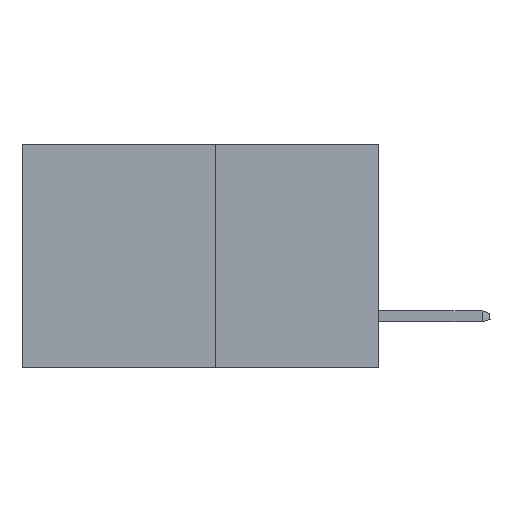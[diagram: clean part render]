
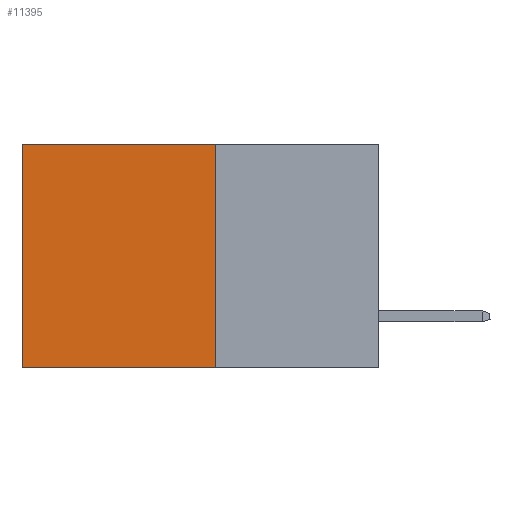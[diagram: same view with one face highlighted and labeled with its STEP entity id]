
A CAD part, left-side view. The second image highlights one B-rep face of the part: STEP entity #11395.
In plain terms, the highlighted planar face has unit normal (-1, 0, 0).
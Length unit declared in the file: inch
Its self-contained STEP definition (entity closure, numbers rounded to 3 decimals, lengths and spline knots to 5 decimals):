
#9 = DIRECTION ( 'NONE',  ( 0., 1., 0. ) ) ;
#455 = CARTESIAN_POINT ( 'NONE',  ( 0.277, 0.27, -0.37 ) ) ;
#3678 = DIRECTION ( 'NONE',  ( 0., 0., -1. ) ) ;
#4418 = LINE ( 'NONE', #22667, #19789 ) ;
#4573 = CARTESIAN_POINT ( 'NONE',  ( 0.277, 0.27, -0.37 ) ) ;
#4858 = LINE ( 'NONE', #13778, #20225 ) ;
#5919 = VECTOR ( 'NONE', #3678, 39.37008 ) ;
#6550 = EDGE_CURVE ( 'NONE', #22512, #9463, #9322, .T. ) ;
#6603 = DIRECTION ( 'NONE',  ( 1., 0., 0. ) ) ;
#7115 = AXIS2_PLACEMENT_3D ( 'NONE', #4573, #6603, #20598 ) ;
#8069 = CARTESIAN_POINT ( 'NONE',  ( 0.277, 0.27, 0. ) ) ;
#8389 = FACE_OUTER_BOUND ( 'NONE', #16503, .T. ) ;
#8718 = VECTOR ( 'NONE', #9, 39.37008 ) ;
#9322 = LINE ( 'NONE', #8069, #8718 ) ;
#9463 = VERTEX_POINT ( 'NONE', #20431 ) ;
#11395 = ADVANCED_FACE ( 'NONE', ( #8389 ), #16656, .F. ) ;
#11755 = EDGE_CURVE ( 'NONE', #9463, #25360, #4858, .T. ) ;
#13001 = ORIENTED_EDGE ( 'NONE', *, *, #14887, .F. ) ;
#13778 = CARTESIAN_POINT ( 'NONE',  ( 0.277, 0.59, -0.37 ) ) ;
#14887 = EDGE_CURVE ( 'NONE', #22512, #19585, #16653, .T. ) ;
#16503 = EDGE_LOOP ( 'NONE', ( #24720, #23755, #13001, #19146 ) ) ;
#16653 = LINE ( 'NONE', #17739, #5919 ) ;
#16656 = PLANE ( 'NONE',  #7115 ) ;
#17739 = CARTESIAN_POINT ( 'NONE',  ( 0.277, 0.27, -0.37 ) ) ;
#19146 = ORIENTED_EDGE ( 'NONE', *, *, #6550, .T. ) ;
#19585 = VERTEX_POINT ( 'NONE', #455 ) ;
#19789 = VECTOR ( 'NONE', #20631, 39.37008 ) ;
#20225 = VECTOR ( 'NONE', #23457, 39.37008 ) ;
#20431 = CARTESIAN_POINT ( 'NONE',  ( 0.277, 0.59, 0. ) ) ;
#20598 = DIRECTION ( 'NONE',  ( 0., 0., -1. ) ) ;
#20631 = DIRECTION ( 'NONE',  ( 0., 1., 0. ) ) ;
#20966 = CARTESIAN_POINT ( 'NONE',  ( 0.277, 0.59, -0.37 ) ) ;
#22067 = CARTESIAN_POINT ( 'NONE',  ( 0.277, 0.27, 0. ) ) ;
#22512 = VERTEX_POINT ( 'NONE', #22067 ) ;
#22667 = CARTESIAN_POINT ( 'NONE',  ( 0.277, 0.27, -0.37 ) ) ;
#22727 = EDGE_CURVE ( 'NONE', #19585, #25360, #4418, .T. ) ;
#23457 = DIRECTION ( 'NONE',  ( 0., 0., -1. ) ) ;
#23755 = ORIENTED_EDGE ( 'NONE', *, *, #22727, .F. ) ;
#24720 = ORIENTED_EDGE ( 'NONE', *, *, #11755, .T. ) ;
#25360 = VERTEX_POINT ( 'NONE', #20966 ) ;
